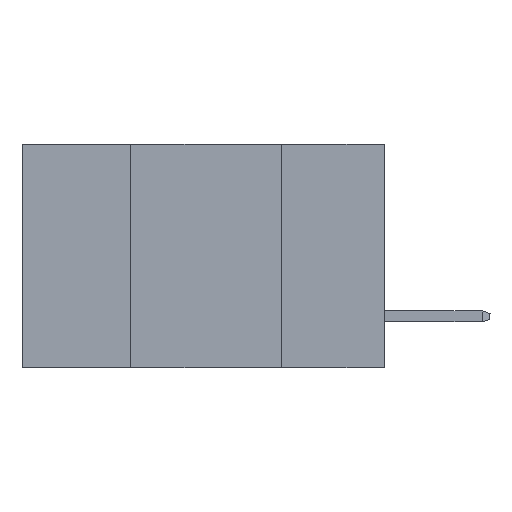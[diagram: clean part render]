
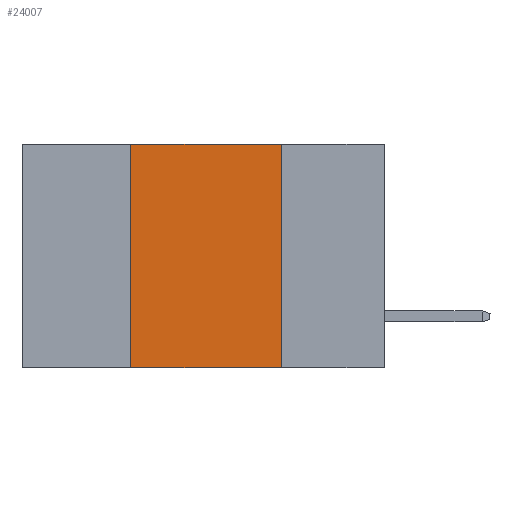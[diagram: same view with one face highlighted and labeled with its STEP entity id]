
A CAD part, left-side view. The second image highlights one B-rep face of the part: STEP entity #24007.
In plain terms, the highlighted planar face has unit normal (-1, 0, 0).
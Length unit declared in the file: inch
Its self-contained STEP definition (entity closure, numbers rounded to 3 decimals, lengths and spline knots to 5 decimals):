
#250 = VERTEX_POINT ( 'NONE', #14452 ) ;
#831 = CARTESIAN_POINT ( 'NONE',  ( 0., 0.17, -0.37 ) ) ;
#1132 = ORIENTED_EDGE ( 'NONE', *, *, #11886, .F. ) ;
#1209 = CARTESIAN_POINT ( 'NONE',  ( 0., 0.6, 0. ) ) ;
#1984 = VECTOR ( 'NONE', #25183, 39.37008 ) ;
#2086 = ORIENTED_EDGE ( 'NONE', *, *, #15784, .F. ) ;
#2564 = ORIENTED_EDGE ( 'NONE', *, *, #17057, .F. ) ;
#3494 = CARTESIAN_POINT ( 'NONE',  ( 0., 0.42, 0. ) ) ;
#3696 = VECTOR ( 'NONE', #8988, 39.37008 ) ;
#4739 = LINE ( 'NONE', #13039, #10737 ) ;
#4759 = VECTOR ( 'NONE', #21604, 39.37008 ) ;
#6266 = EDGE_LOOP ( 'NONE', ( #2564, #1132, #2086, #18134 ) ) ;
#6599 = DIRECTION ( 'NONE',  ( 0., -1., 0. ) ) ;
#8988 = DIRECTION ( 'NONE',  ( 0., 0., -1. ) ) ;
#9243 = DIRECTION ( 'NONE',  ( 0., 0., -1. ) ) ;
#10737 = VECTOR ( 'NONE', #6599, 39.37008 ) ;
#11205 = PLANE ( 'NONE',  #16872 ) ;
#11856 = VERTEX_POINT ( 'NONE', #16502 ) ;
#11886 = EDGE_CURVE ( 'NONE', #13392, #11856, #17176, .T. ) ;
#13039 = CARTESIAN_POINT ( 'NONE',  ( 0., 0.6, -0.37 ) ) ;
#13296 = LINE ( 'NONE', #17206, #1984 ) ;
#13392 = VERTEX_POINT ( 'NONE', #3494 ) ;
#13744 = VERTEX_POINT ( 'NONE', #15161 ) ;
#14119 = EDGE_CURVE ( 'NONE', #13744, #250, #4739, .T. ) ;
#14452 = CARTESIAN_POINT ( 'NONE',  ( 0., 0.17, -0.37 ) ) ;
#14510 = DIRECTION ( 'NONE',  ( 1., 0., 0. ) ) ;
#15161 = CARTESIAN_POINT ( 'NONE',  ( 0., 0.42, -0.37 ) ) ;
#15784 = EDGE_CURVE ( 'NONE', #13744, #13392, #13296, .T. ) ;
#16502 = CARTESIAN_POINT ( 'NONE',  ( 0., 0.17, 0. ) ) ;
#16872 = AXIS2_PLACEMENT_3D ( 'NONE', #1209, #14510, #9243 ) ;
#17057 = EDGE_CURVE ( 'NONE', #11856, #250, #20750, .T. ) ;
#17176 = LINE ( 'NONE', #23176, #4759 ) ;
#17206 = CARTESIAN_POINT ( 'NONE',  ( 0., 0.42, -0.37 ) ) ;
#18134 = ORIENTED_EDGE ( 'NONE', *, *, #14119, .T. ) ;
#19294 = FACE_OUTER_BOUND ( 'NONE', #6266, .T. ) ;
#20750 = LINE ( 'NONE', #831, #3696 ) ;
#21604 = DIRECTION ( 'NONE',  ( 0., -1., 0. ) ) ;
#23176 = CARTESIAN_POINT ( 'NONE',  ( 0., 0.6, 0. ) ) ;
#24007 = ADVANCED_FACE ( 'NONE', ( #19294 ), #11205, .F. ) ;
#25183 = DIRECTION ( 'NONE',  ( 0., 0., 1. ) ) ;
